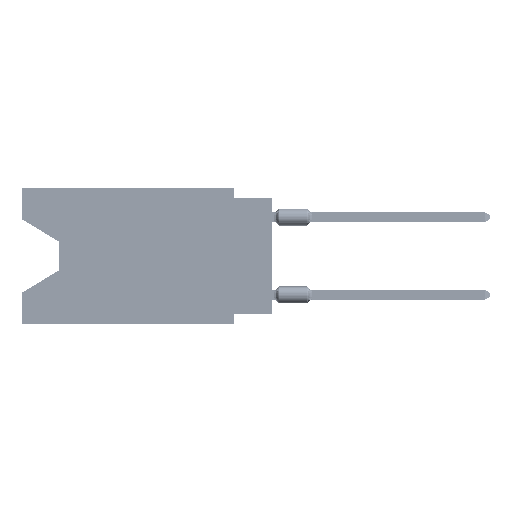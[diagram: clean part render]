
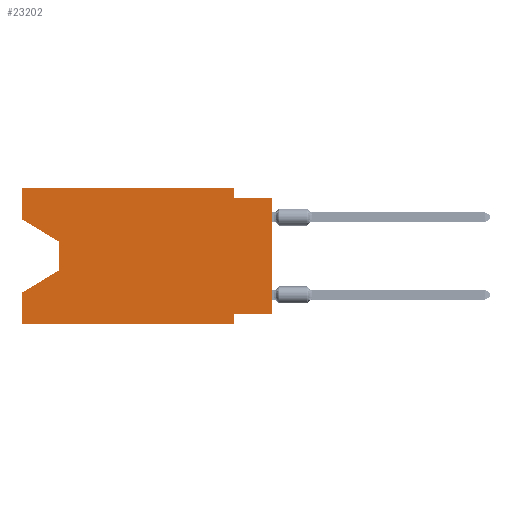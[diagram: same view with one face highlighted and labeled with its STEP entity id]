
A CAD part, left-side view. The second image highlights one B-rep face of the part: STEP entity #23202.
In plain terms, the highlighted planar face has unit normal (-1, 0, 0).
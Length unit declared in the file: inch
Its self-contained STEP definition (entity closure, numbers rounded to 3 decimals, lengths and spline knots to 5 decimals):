
#231 = VERTEX_POINT ( 'NONE', #121626 ) ;
#1302 = VERTEX_POINT ( 'NONE', #20873 ) ;
#2335 = LINE ( 'NONE', #88525, #76172 ) ;
#6224 = ORIENTED_EDGE ( 'NONE', *, *, #58393, .T. ) ;
#7407 = ORIENTED_EDGE ( 'NONE', *, *, #19701, .T. ) ;
#7425 = DIRECTION ( 'NONE',  ( 0., -1., 0. ) ) ;
#7665 = VERTEX_POINT ( 'NONE', #45753 ) ;
#10745 = VERTEX_POINT ( 'NONE', #15552 ) ;
#11526 = CARTESIAN_POINT ( 'NONE',  ( 0., 0.1, 0. ) ) ;
#13454 = VECTOR ( 'NONE', #39829, 39.37008 ) ;
#13847 = EDGE_CURVE ( 'NONE', #21515, #1302, #66065, .T. ) ;
#15552 = CARTESIAN_POINT ( 'NONE',  ( 0., 0.1, -0.025 ) ) ;
#16003 = CARTESIAN_POINT ( 'NONE',  ( 0., 0., -0.325 ) ) ;
#16153 = ORIENTED_EDGE ( 'NONE', *, *, #50737, .T. ) ;
#16679 = LINE ( 'NONE', #83204, #77160 ) ;
#18573 = VECTOR ( 'NONE', #24633, 39.37008 ) ;
#18896 = VERTEX_POINT ( 'NONE', #96188 ) ;
#18938 = CARTESIAN_POINT ( 'NONE',  ( 0., 0.55, -0.212 ) ) ;
#19234 = VECTOR ( 'NONE', #99372, 39.37008 ) ;
#19701 = EDGE_CURVE ( 'NONE', #7665, #18896, #33465, .T. ) ;
#20873 = CARTESIAN_POINT ( 'NONE',  ( 0., 0.645, -0.26975 ) ) ;
#21515 = VERTEX_POINT ( 'NONE', #118350 ) ;
#21624 = EDGE_CURVE ( 'NONE', #78974, #29901, #16679, .T. ) ;
#22998 = DIRECTION ( 'NONE',  ( 0., 0., 1. ) ) ;
#23032 = LINE ( 'NONE', #118519, #37445 ) ;
#23202 = ADVANCED_FACE ( 'NONE', ( #97528 ), #96920, .F. ) ;
#24633 = DIRECTION ( 'NONE',  ( 0., 1., 0. ) ) ;
#28562 = VECTOR ( 'NONE', #90509, 39.37008 ) ;
#28694 = EDGE_CURVE ( 'NONE', #231, #113321, #114999, .T. ) ;
#29038 = CARTESIAN_POINT ( 'NONE',  ( 0., 0.1, -0.35 ) ) ;
#29155 = VERTEX_POINT ( 'NONE', #95161 ) ;
#29901 = VERTEX_POINT ( 'NONE', #11526 ) ;
#30939 = CARTESIAN_POINT ( 'NONE',  ( 0., 0.55, -0.138 ) ) ;
#31612 = CARTESIAN_POINT ( 'NONE',  ( 0., 0.645, 0. ) ) ;
#32542 = ORIENTED_EDGE ( 'NONE', *, *, #52426, .T. ) ;
#32861 = CARTESIAN_POINT ( 'NONE',  ( 0., 0., 0. ) ) ;
#33465 = LINE ( 'NONE', #32861, #116211 ) ;
#33467 = CARTESIAN_POINT ( 'NONE',  ( 0., 0., -0.025 ) ) ;
#35080 = CARTESIAN_POINT ( 'NONE',  ( 0., 0.55, -0.138 ) ) ;
#36318 = ORIENTED_EDGE ( 'NONE', *, *, #28694, .F. ) ;
#36720 = VECTOR ( 'NONE', #105547, 39.37008 ) ;
#37445 = VECTOR ( 'NONE', #61834, 39.37008 ) ;
#37820 = CARTESIAN_POINT ( 'NONE',  ( 0., 0.1, 0. ) ) ;
#38959 = DIRECTION ( 'NONE',  ( 0., 0., 1. ) ) ;
#39445 = LINE ( 'NONE', #88652, #77840 ) ;
#39829 = DIRECTION ( 'NONE',  ( 0., 0., -1. ) ) ;
#45753 = CARTESIAN_POINT ( 'NONE',  ( 0., 0., -0.325 ) ) ;
#47479 = EDGE_CURVE ( 'NONE', #7665, #231, #78871, .T. ) ;
#48470 = CARTESIAN_POINT ( 'NONE',  ( 0., 0.1, -0.35 ) ) ;
#50737 = EDGE_CURVE ( 'NONE', #29155, #88076, #39445, .T. ) ;
#51626 = VECTOR ( 'NONE', #84245, 39.37008 ) ;
#52074 = ORIENTED_EDGE ( 'NONE', *, *, #13847, .F. ) ;
#52426 = EDGE_CURVE ( 'NONE', #21515, #113321, #2335, .T. ) ;
#53836 = EDGE_LOOP ( 'NONE', ( #16153, #6224, #74236, #52074, #32542, #36318, #118135, #7407, #83408, #87754, #81765, #96490 ) ) ;
#58157 = DIRECTION ( 'NONE',  ( 1., 0., 0. ) ) ;
#58393 = EDGE_CURVE ( 'NONE', #88076, #105030, #73249, .T. ) ;
#61834 = DIRECTION ( 'NONE',  ( 0., 0., 1. ) ) ;
#61962 = CARTESIAN_POINT ( 'NONE',  ( 0., 0.645, 0. ) ) ;
#62878 = EDGE_CURVE ( 'NONE', #10745, #18896, #117873, .T. ) ;
#66065 = LINE ( 'NONE', #103654, #66157 ) ;
#66157 = VECTOR ( 'NONE', #38959, 39.37008 ) ;
#70340 = EDGE_CURVE ( 'NONE', #29155, #78974, #23032, .T. ) ;
#73249 = LINE ( 'NONE', #35080, #28562 ) ;
#74236 = ORIENTED_EDGE ( 'NONE', *, *, #103369, .T. ) ;
#76172 = VECTOR ( 'NONE', #95379, 39.37008 ) ;
#76624 = DIRECTION ( 'NONE',  ( 0., 0., -1. ) ) ;
#77160 = VECTOR ( 'NONE', #7425, 39.37008 ) ;
#77840 = VECTOR ( 'NONE', #104760, 39.37008 ) ;
#78871 = LINE ( 'NONE', #16003, #18573 ) ;
#78974 = VERTEX_POINT ( 'NONE', #61962 ) ;
#81765 = ORIENTED_EDGE ( 'NONE', *, *, #21624, .F. ) ;
#83204 = CARTESIAN_POINT ( 'NONE',  ( 0., 0.645, 0. ) ) ;
#83408 = ORIENTED_EDGE ( 'NONE', *, *, #62878, .F. ) ;
#84245 = DIRECTION ( 'NONE',  ( 0., 0.855, -0.519 ) ) ;
#87754 = ORIENTED_EDGE ( 'NONE', *, *, #116849, .F. ) ;
#88076 = VERTEX_POINT ( 'NONE', #30939 ) ;
#88525 = CARTESIAN_POINT ( 'NONE',  ( 0., 0.645, -0.35 ) ) ;
#88652 = CARTESIAN_POINT ( 'NONE',  ( 0., 0.645, -0.08025 ) ) ;
#89558 = CARTESIAN_POINT ( 'NONE',  ( 0., 0.55, -0.212 ) ) ;
#90509 = DIRECTION ( 'NONE',  ( 0., 0., -1. ) ) ;
#93483 = LINE ( 'NONE', #18938, #51626 ) ;
#95161 = CARTESIAN_POINT ( 'NONE',  ( 0., 0.645, -0.08025 ) ) ;
#95379 = DIRECTION ( 'NONE',  ( 0., -1., 0. ) ) ;
#96188 = CARTESIAN_POINT ( 'NONE',  ( 0., 0., -0.025 ) ) ;
#96290 = LINE ( 'NONE', #37820, #36720 ) ;
#96490 = ORIENTED_EDGE ( 'NONE', *, *, #70340, .F. ) ;
#96920 = PLANE ( 'NONE',  #100376 ) ;
#97528 = FACE_OUTER_BOUND ( 'NONE', #53836, .T. ) ;
#99372 = DIRECTION ( 'NONE',  ( 0., -1., 0. ) ) ;
#100376 = AXIS2_PLACEMENT_3D ( 'NONE', #31612, #58157, #76624 ) ;
#103369 = EDGE_CURVE ( 'NONE', #105030, #1302, #93483, .T. ) ;
#103654 = CARTESIAN_POINT ( 'NONE',  ( 0., 0.645, 0. ) ) ;
#104760 = DIRECTION ( 'NONE',  ( 0., -0.855, -0.519 ) ) ;
#105030 = VERTEX_POINT ( 'NONE', #89558 ) ;
#105547 = DIRECTION ( 'NONE',  ( 0., 0., -1. ) ) ;
#113321 = VERTEX_POINT ( 'NONE', #29038 ) ;
#114999 = LINE ( 'NONE', #48470, #13454 ) ;
#116211 = VECTOR ( 'NONE', #22998, 39.37008 ) ;
#116849 = EDGE_CURVE ( 'NONE', #29901, #10745, #96290, .T. ) ;
#117873 = LINE ( 'NONE', #33467, #19234 ) ;
#118135 = ORIENTED_EDGE ( 'NONE', *, *, #47479, .F. ) ;
#118350 = CARTESIAN_POINT ( 'NONE',  ( 0., 0.645, -0.35 ) ) ;
#118519 = CARTESIAN_POINT ( 'NONE',  ( 0., 0.645, 0. ) ) ;
#121626 = CARTESIAN_POINT ( 'NONE',  ( 0., 0.1, -0.325 ) ) ;
